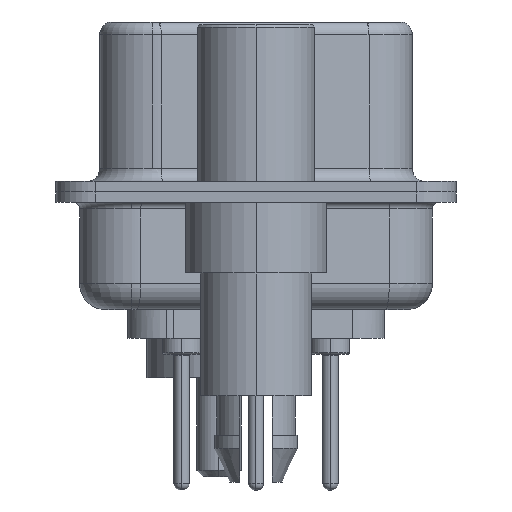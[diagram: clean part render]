
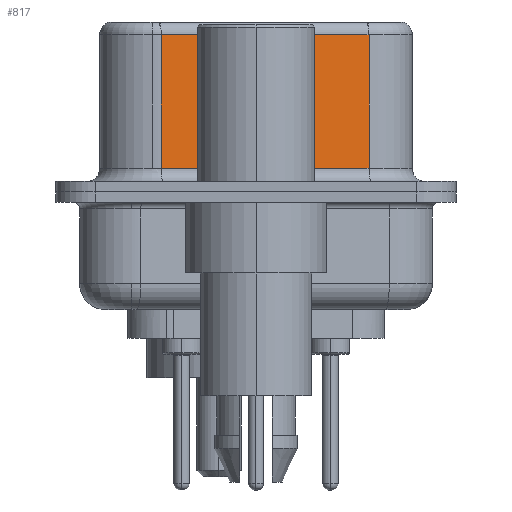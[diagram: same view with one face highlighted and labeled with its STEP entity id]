
A CAD part, left-side view. The second image highlights one B-rep face of the part: STEP entity #817.
In plain terms, the highlighted planar face has unit normal (-0.985, -0.174, 0).
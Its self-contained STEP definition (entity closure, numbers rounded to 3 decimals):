
#817 = ADVANCED_FACE ( 'NONE', ( #1155 ), #17093, .F. ) ;
#1155 = FACE_OUTER_BOUND ( 'NONE', #11499, .T. ) ;
#3157 = CARTESIAN_POINT ( 'NONE',  ( 5.132, -4.322, 6.02 ) ) ;
#3391 = CARTESIAN_POINT ( 'NONE',  ( 5.132, -4.322, 0.9 ) ) ;
#4425 = ORIENTED_EDGE ( 'NONE', *, *, #12286, .T. ) ;
#5301 = EDGE_CURVE ( 'NONE', #29672, #7715, #20269, .T. ) ;
#6507 = EDGE_CURVE ( 'NONE', #26469, #7715, #23747, .T. ) ;
#6662 = ORIENTED_EDGE ( 'NONE', *, *, #5301, .T. ) ;
#6848 = CARTESIAN_POINT ( 'NONE',  ( 5.132, -4.322, 0.9 ) ) ;
#7715 = VERTEX_POINT ( 'NONE', #6848 ) ;
#9666 = CARTESIAN_POINT ( 'NONE',  ( 5.132, -4.322, 6.52 ) ) ;
#9745 = VECTOR ( 'NONE', #29428, 1000. ) ;
#10186 = DIRECTION ( 'NONE',  ( 0., 0., -1. ) ) ;
#10489 = CARTESIAN_POINT ( 'NONE',  ( 5.132, -4.322, 6.02 ) ) ;
#11392 = DIRECTION ( 'NONE',  ( -0.174, 0.985, 0. ) ) ;
#11499 = EDGE_LOOP ( 'NONE', ( #12007, #4425, #21645, #6662 ) ) ;
#12007 = ORIENTED_EDGE ( 'NONE', *, *, #6507, .F. ) ;
#12286 = EDGE_CURVE ( 'NONE', #26469, #20871, #23060, .T. ) ;
#13308 = DIRECTION ( 'NONE',  ( 0.174, -0.985, 0. ) ) ;
#13703 = VECTOR ( 'NONE', #13308, 1000. ) ;
#14850 = CARTESIAN_POINT ( 'NONE',  ( 5.132, -4.322, 6.52 ) ) ;
#16401 = VECTOR ( 'NONE', #17916, 1000. ) ;
#17093 = PLANE ( 'NONE',  #29781 ) ;
#17916 = DIRECTION ( 'NONE',  ( -0.174, 0.985, 0. ) ) ;
#20269 = LINE ( 'NONE', #3391, #13703 ) ;
#20871 = VERTEX_POINT ( 'NONE', #23119 ) ;
#21433 = DIRECTION ( 'NONE',  ( 0.985, 0.174, 0. ) ) ;
#21645 = ORIENTED_EDGE ( 'NONE', *, *, #24961, .T. ) ;
#22955 = VECTOR ( 'NONE', #10186, 1000. ) ;
#23060 = LINE ( 'NONE', #3157, #16401 ) ;
#23119 = CARTESIAN_POINT ( 'NONE',  ( 3.73, 3.628, 6.02 ) ) ;
#23747 = LINE ( 'NONE', #9666, #22955 ) ;
#24961 = EDGE_CURVE ( 'NONE', #20871, #29672, #29494, .T. ) ;
#26469 = VERTEX_POINT ( 'NONE', #10489 ) ;
#26954 = CARTESIAN_POINT ( 'NONE',  ( 3.73, 3.628, 6.52 ) ) ;
#27853 = CARTESIAN_POINT ( 'NONE',  ( 3.73, 3.628, 0.9 ) ) ;
#29428 = DIRECTION ( 'NONE',  ( 0., 0., -1. ) ) ;
#29494 = LINE ( 'NONE', #26954, #9745 ) ;
#29672 = VERTEX_POINT ( 'NONE', #27853 ) ;
#29781 = AXIS2_PLACEMENT_3D ( 'NONE', #14850, #21433, #11392 ) ;
